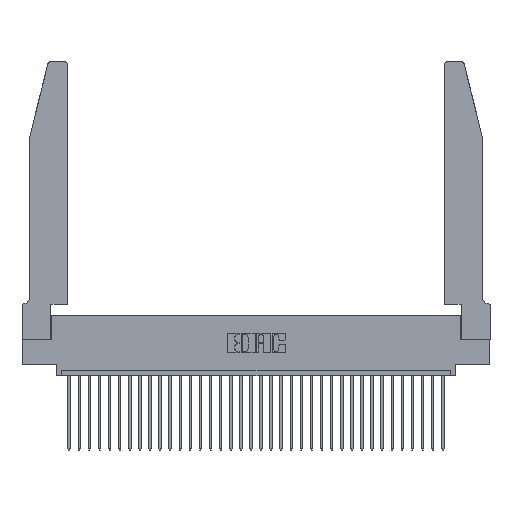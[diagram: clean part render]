
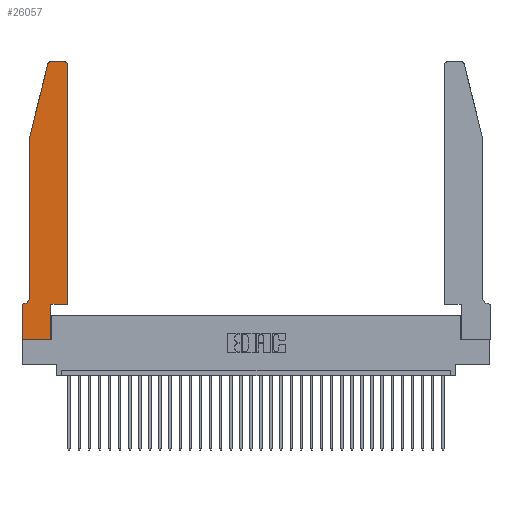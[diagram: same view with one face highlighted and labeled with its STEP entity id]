
A CAD part, top view. The second image highlights one B-rep face of the part: STEP entity #26057.
In plain terms, the highlighted planar face has unit normal (0, 0, 1).
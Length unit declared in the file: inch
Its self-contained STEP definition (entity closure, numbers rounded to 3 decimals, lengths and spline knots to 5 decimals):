
#243 = CARTESIAN_POINT ( 'NONE',  ( 0.0755, 2., 0.37 ) ) ;
#297 = EDGE_CURVE ( 'NONE', #9554, #10879, #33926, .T. ) ;
#1400 = CARTESIAN_POINT ( 'NONE',  ( 0.4505, 0.35, 0.37 ) ) ;
#1717 = ORIENTED_EDGE ( 'NONE', *, *, #21427, .T. ) ;
#2380 = VECTOR ( 'NONE', #12783, 39.37008 ) ;
#2509 = VERTEX_POINT ( 'NONE', #9827 ) ;
#2777 = CIRCLE ( 'NONE', #14173, 0.07 ) ;
#3067 = EDGE_CURVE ( 'NONE', #27668, #13212, #20653, .T. ) ;
#3332 = VERTEX_POINT ( 'NONE', #6375 ) ;
#3455 = LINE ( 'NONE', #24966, #15875 ) ;
#4253 = CARTESIAN_POINT ( 'NONE',  ( 0.284, 2.75, 0.37 ) ) ;
#4316 = DIRECTION ( 'NONE',  ( 0., -1., 0. ) ) ;
#4627 = CARTESIAN_POINT ( 'NONE',  ( 0.2605, 2.75, 0.37 ) ) ;
#5056 = VECTOR ( 'NONE', #4316, 39.37008 ) ;
#6375 = CARTESIAN_POINT ( 'NONE',  ( 0.2865, 0.35, 0.37 ) ) ;
#7983 = EDGE_CURVE ( 'NONE', #29836, #9554, #28489, .T. ) ;
#9112 = EDGE_CURVE ( 'NONE', #15819, #27290, #2777, .T. ) ;
#9153 = LINE ( 'NONE', #4627, #27046 ) ;
#9399 = DIRECTION ( 'NONE',  ( 0., 0., 1. ) ) ;
#9554 = VERTEX_POINT ( 'NONE', #14260 ) ;
#9827 = CARTESIAN_POINT ( 'NONE',  ( 0.4505, 2.72, 0.37 ) ) ;
#9901 = VERTEX_POINT ( 'NONE', #24975 ) ;
#9922 = DIRECTION ( 'NONE',  ( 1., 0., 0. ) ) ;
#10042 = CARTESIAN_POINT ( 'NONE',  ( 0.4205, 2.72, 0.37 ) ) ;
#10879 = VERTEX_POINT ( 'NONE', #19641 ) ;
#11220 = LINE ( 'NONE', #19215, #16549 ) ;
#11240 = ORIENTED_EDGE ( 'NONE', *, *, #11288, .T. ) ;
#11288 = EDGE_CURVE ( 'NONE', #27290, #27668, #3455, .T. ) ;
#12202 = VECTOR ( 'NONE', #14988, 39.37008 ) ;
#12783 = DIRECTION ( 'NONE',  ( 1., 0., 0. ) ) ;
#12960 = ORIENTED_EDGE ( 'NONE', *, *, #297, .T. ) ;
#13212 = VERTEX_POINT ( 'NONE', #16992 ) ;
#13656 = EDGE_CURVE ( 'NONE', #16314, #3332, #29146, .T. ) ;
#14173 = AXIS2_PLACEMENT_3D ( 'NONE', #28529, #28949, #23502 ) ;
#14192 = EDGE_LOOP ( 'NONE', ( #31389, #21644, #12960, #25641, #33840, #11240, #14810, #21393, #28469, #28951, #15147, #1717 ) ) ;
#14260 = CARTESIAN_POINT ( 'NONE',  ( 0.25487, 2.72718, 0.37 ) ) ;
#14341 = DIRECTION ( 'NONE',  ( 0., 1., 0. ) ) ;
#14810 = ORIENTED_EDGE ( 'NONE', *, *, #3067, .T. ) ;
#14972 = VECTOR ( 'NONE', #32772, 39.37008 ) ;
#14988 = DIRECTION ( 'NONE',  ( -0.239, -0.971, 0. ) ) ;
#14991 = FACE_OUTER_BOUND ( 'NONE', #14192, .T. ) ;
#15026 = DIRECTION ( 'NONE',  ( -1., 0., 0. ) ) ;
#15147 = ORIENTED_EDGE ( 'NONE', *, *, #33013, .T. ) ;
#15645 = CARTESIAN_POINT ( 'NONE',  ( 0., 0., 0.37 ) ) ;
#15666 = CARTESIAN_POINT ( 'NONE',  ( 0.284, 2.72, 0.37 ) ) ;
#15710 = CARTESIAN_POINT ( 'NONE',  ( 0.4505, 0.35, 0.37 ) ) ;
#15819 = VERTEX_POINT ( 'NONE', #24871 ) ;
#15875 = VECTOR ( 'NONE', #15026, 39.37008 ) ;
#15907 = EDGE_CURVE ( 'NONE', #13212, #16314, #23352, .T. ) ;
#16314 = VERTEX_POINT ( 'NONE', #17601 ) ;
#16549 = VECTOR ( 'NONE', #27104, 39.37008 ) ;
#16992 = CARTESIAN_POINT ( 'NONE',  ( 0., 0., 0.37 ) ) ;
#17601 = CARTESIAN_POINT ( 'NONE',  ( 0.2865, 0., 0.37 ) ) ;
#18611 = LINE ( 'NONE', #19811, #14972 ) ;
#18731 = DIRECTION ( 'NONE',  ( 0., 0., 1. ) ) ;
#18906 = VECTOR ( 'NONE', #22569, 39.37008 ) ;
#19215 = CARTESIAN_POINT ( 'NONE',  ( 0.0755, 2., 0.37 ) ) ;
#19641 = CARTESIAN_POINT ( 'NONE',  ( 0.0755, 2., 0.37 ) ) ;
#19811 = CARTESIAN_POINT ( 'NONE',  ( 0.4505, 0.35, 0.37 ) ) ;
#19934 = CARTESIAN_POINT ( 'NONE',  ( 0.2865, 0.35, 0.37 ) ) ;
#20062 = DIRECTION ( 'NONE',  ( 0., 0., 1. ) ) ;
#20253 = VECTOR ( 'NONE', #14341, 39.37008 ) ;
#20653 = LINE ( 'NONE', #22435, #5056 ) ;
#21393 = ORIENTED_EDGE ( 'NONE', *, *, #15907, .T. ) ;
#21427 = EDGE_CURVE ( 'NONE', #2509, #9901, #25471, .T. ) ;
#21510 = EDGE_CURVE ( 'NONE', #9901, #29836, #9153, .T. ) ;
#21644 = ORIENTED_EDGE ( 'NONE', *, *, #7983, .T. ) ;
#22268 = CARTESIAN_POINT ( 'NONE',  ( 0., 0.35, 0.37 ) ) ;
#22435 = CARTESIAN_POINT ( 'NONE',  ( 0., 0., 0.37 ) ) ;
#22569 = DIRECTION ( 'NONE',  ( 0., 1., 0. ) ) ;
#22727 = AXIS2_PLACEMENT_3D ( 'NONE', #22268, #9399, #29953 ) ;
#23352 = LINE ( 'NONE', #15645, #2380 ) ;
#23502 = DIRECTION ( 'NONE',  ( -1., 0., 0. ) ) ;
#23791 = AXIS2_PLACEMENT_3D ( 'NONE', #15666, #18731, #30754 ) ;
#23824 = CARTESIAN_POINT ( 'NONE',  ( 0., 0.35, 0.37 ) ) ;
#24871 = CARTESIAN_POINT ( 'NONE',  ( 0.0755, 0.42, 0.37 ) ) ;
#24966 = CARTESIAN_POINT ( 'NONE',  ( 0.0755, 0.35, 0.37 ) ) ;
#24975 = CARTESIAN_POINT ( 'NONE',  ( 0.4205, 2.75, 0.37 ) ) ;
#25471 = CIRCLE ( 'NONE', #32958, 0.03 ) ;
#25567 = LINE ( 'NONE', #1400, #20253 ) ;
#25641 = ORIENTED_EDGE ( 'NONE', *, *, #27837, .T. ) ;
#25821 = VERTEX_POINT ( 'NONE', #15710 ) ;
#26057 = ADVANCED_FACE ( 'NONE', ( #14991 ), #30406, .T. ) ;
#27046 = VECTOR ( 'NONE', #33863, 39.37008 ) ;
#27104 = DIRECTION ( 'NONE',  ( 0., -1., 0. ) ) ;
#27273 = EDGE_CURVE ( 'NONE', #3332, #25821, #18611, .T. ) ;
#27290 = VERTEX_POINT ( 'NONE', #27705 ) ;
#27668 = VERTEX_POINT ( 'NONE', #23824 ) ;
#27705 = CARTESIAN_POINT ( 'NONE',  ( 0.0055, 0.35, 0.37 ) ) ;
#27837 = EDGE_CURVE ( 'NONE', #10879, #15819, #11220, .T. ) ;
#28469 = ORIENTED_EDGE ( 'NONE', *, *, #13656, .T. ) ;
#28489 = CIRCLE ( 'NONE', #23791, 0.03 ) ;
#28529 = CARTESIAN_POINT ( 'NONE',  ( 0.0055, 0.42, 0.37 ) ) ;
#28949 = DIRECTION ( 'NONE',  ( 0., 0., -1. ) ) ;
#28951 = ORIENTED_EDGE ( 'NONE', *, *, #27273, .T. ) ;
#29146 = LINE ( 'NONE', #19934, #18906 ) ;
#29836 = VERTEX_POINT ( 'NONE', #4253 ) ;
#29953 = DIRECTION ( 'NONE',  ( 1., 0., 0. ) ) ;
#30406 = PLANE ( 'NONE',  #22727 ) ;
#30754 = DIRECTION ( 'NONE',  ( 1., 0., 0. ) ) ;
#31389 = ORIENTED_EDGE ( 'NONE', *, *, #21510, .T. ) ;
#32772 = DIRECTION ( 'NONE',  ( 1., 0., 0. ) ) ;
#32958 = AXIS2_PLACEMENT_3D ( 'NONE', #10042, #20062, #9922 ) ;
#33013 = EDGE_CURVE ( 'NONE', #25821, #2509, #25567, .T. ) ;
#33840 = ORIENTED_EDGE ( 'NONE', *, *, #9112, .T. ) ;
#33863 = DIRECTION ( 'NONE',  ( -1., 0., 0. ) ) ;
#33926 = LINE ( 'NONE', #243, #12202 ) ;
